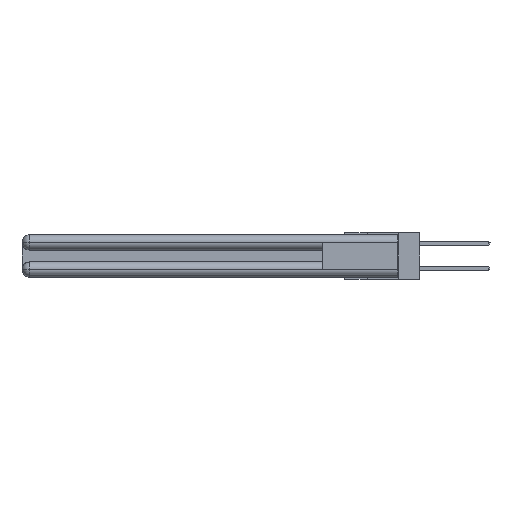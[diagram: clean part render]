
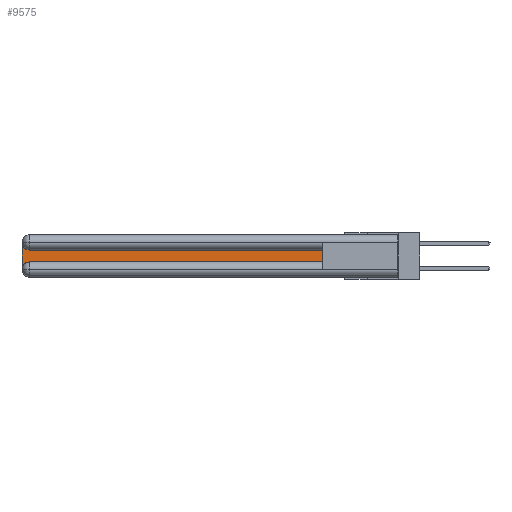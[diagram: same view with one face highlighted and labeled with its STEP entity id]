
A CAD part, left-side view. The second image highlights one B-rep face of the part: STEP entity #9575.
In plain terms, the highlighted planar face has unit normal (-1, 0, 0).
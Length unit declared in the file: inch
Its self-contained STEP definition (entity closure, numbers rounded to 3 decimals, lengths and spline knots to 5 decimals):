
#377 = AXIS2_PLACEMENT_3D ( 'NONE', #25175, #944, #1402 ) ;
#628 = ORIENTED_EDGE ( 'NONE', *, *, #34656, .T. ) ;
#944 = DIRECTION ( 'NONE',  ( 1., 0., 0. ) ) ;
#1146 = VECTOR ( 'NONE', #25405, 39.37008 ) ;
#1335 = CARTESIAN_POINT ( 'NONE',  ( 0.075, 2.94, -0.2775 ) ) ;
#1402 = DIRECTION ( 'NONE',  ( 0., 0., -1. ) ) ;
#1623 = VERTEX_POINT ( 'NONE', #31044 ) ;
#1695 = CARTESIAN_POINT ( 'NONE',  ( 0.075, 3., -0.1225 ) ) ;
#2737 = DIRECTION ( 'NONE',  ( 0., 0., 1. ) ) ;
#3127 = CIRCLE ( 'NONE', #15570, 0.06 ) ;
#3439 = VERTEX_POINT ( 'NONE', #27509 ) ;
#3770 = VECTOR ( 'NONE', #30139, 39.37008 ) ;
#5044 = VERTEX_POINT ( 'NONE', #26700 ) ;
#5486 = VECTOR ( 'NONE', #2737, 39.37008 ) ;
#5614 = EDGE_CURVE ( 'NONE', #15825, #28669, #15600, .T. ) ;
#5916 = ORIENTED_EDGE ( 'NONE', *, *, #10511, .T. ) ;
#6031 = CIRCLE ( 'NONE', #377, 0.06 ) ;
#6592 = CARTESIAN_POINT ( 'NONE',  ( 0.075, 0.6, -0.1225 ) ) ;
#9256 = ORIENTED_EDGE ( 'NONE', *, *, #5614, .T. ) ;
#9575 = ADVANCED_FACE ( 'NONE', ( #11415 ), #18050, .F. ) ;
#10511 = EDGE_CURVE ( 'NONE', #21408, #1623, #28570, .T. ) ;
#11415 = FACE_OUTER_BOUND ( 'NONE', #23262, .T. ) ;
#13304 = LINE ( 'NONE', #6592, #1146 ) ;
#15570 = AXIS2_PLACEMENT_3D ( 'NONE', #1335, #33687, #20162 ) ;
#15600 = LINE ( 'NONE', #33410, #27374 ) ;
#15825 = VERTEX_POINT ( 'NONE', #33316 ) ;
#16381 = CARTESIAN_POINT ( 'NONE',  ( 0.075, 0.6, -0.2175 ) ) ;
#16912 = CARTESIAN_POINT ( 'NONE',  ( 0.075, 3., -0.2175 ) ) ;
#17590 = DIRECTION ( 'NONE',  ( 0., 0., -1. ) ) ;
#18034 = AXIS2_PLACEMENT_3D ( 'NONE', #1695, #22859, #17590 ) ;
#18050 = PLANE ( 'NONE',  #18034 ) ;
#20162 = DIRECTION ( 'NONE',  ( 0., 0., -1. ) ) ;
#20210 = DIRECTION ( 'NONE',  ( 0., -1., 0. ) ) ;
#21408 = VERTEX_POINT ( 'NONE', #32080 ) ;
#21692 = ORIENTED_EDGE ( 'NONE', *, *, #28303, .T. ) ;
#22048 = ORIENTED_EDGE ( 'NONE', *, *, #31806, .T. ) ;
#22859 = DIRECTION ( 'NONE',  ( 1., 0., 0. ) ) ;
#23262 = EDGE_LOOP ( 'NONE', ( #21692, #33216, #5916, #628, #9256, #22048 ) ) ;
#25175 = CARTESIAN_POINT ( 'NONE',  ( 0.075, 2.94, -0.0625 ) ) ;
#25405 = DIRECTION ( 'NONE',  ( 0., 1., 0. ) ) ;
#26700 = CARTESIAN_POINT ( 'NONE',  ( 0.075, 2.94, -0.1225 ) ) ;
#27374 = VECTOR ( 'NONE', #20210, 39.37008 ) ;
#27509 = CARTESIAN_POINT ( 'NONE',  ( 0.075, 0.6, -0.1225 ) ) ;
#28303 = EDGE_CURVE ( 'NONE', #3439, #5044, #13304, .T. ) ;
#28570 = LINE ( 'NONE', #16912, #3770 ) ;
#28669 = VERTEX_POINT ( 'NONE', #31676 ) ;
#30139 = DIRECTION ( 'NONE',  ( 0., 0., -1. ) ) ;
#30424 = EDGE_CURVE ( 'NONE', #5044, #21408, #6031, .T. ) ;
#31044 = CARTESIAN_POINT ( 'NONE',  ( 0.075, 3., -0.2775 ) ) ;
#31676 = CARTESIAN_POINT ( 'NONE',  ( 0.075, 0.6, -0.2175 ) ) ;
#31806 = EDGE_CURVE ( 'NONE', #28669, #3439, #34024, .T. ) ;
#32080 = CARTESIAN_POINT ( 'NONE',  ( 0.075, 3., -0.0625 ) ) ;
#33216 = ORIENTED_EDGE ( 'NONE', *, *, #30424, .T. ) ;
#33316 = CARTESIAN_POINT ( 'NONE',  ( 0.075, 2.94, -0.2175 ) ) ;
#33410 = CARTESIAN_POINT ( 'NONE',  ( 0.075, 0.6, -0.2175 ) ) ;
#33687 = DIRECTION ( 'NONE',  ( 1., 0., 0. ) ) ;
#34024 = LINE ( 'NONE', #16381, #5486 ) ;
#34656 = EDGE_CURVE ( 'NONE', #1623, #15825, #3127, .T. ) ;
